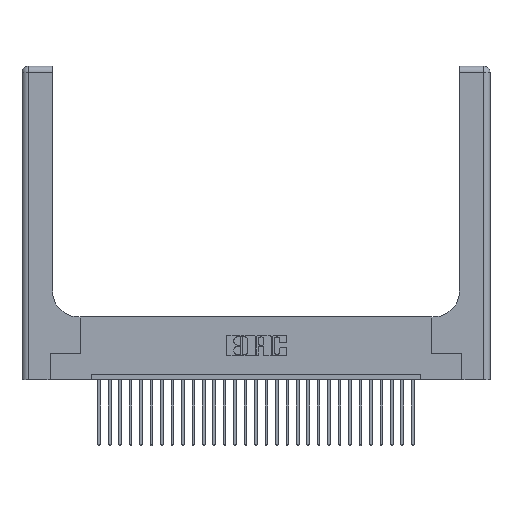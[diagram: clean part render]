
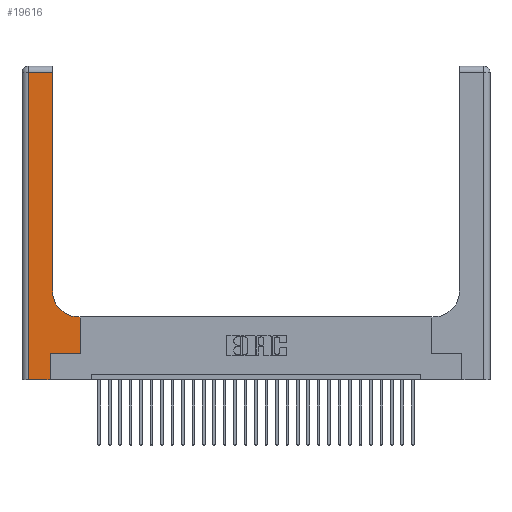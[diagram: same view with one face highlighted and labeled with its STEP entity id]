
A CAD part, top view. The second image highlights one B-rep face of the part: STEP entity #19616.
In plain terms, the highlighted planar face has unit normal (0, 0, 1).
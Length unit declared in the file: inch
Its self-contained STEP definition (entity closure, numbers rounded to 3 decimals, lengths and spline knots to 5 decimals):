
#336 = PLANE ( 'NONE',  #2996 ) ;
#533 = CARTESIAN_POINT ( 'NONE',  ( 0., 3., 0.37 ) ) ;
#578 = VERTEX_POINT ( 'NONE', #17617 ) ;
#620 = FACE_OUTER_BOUND ( 'NONE', #22212, .T. ) ;
#878 = CARTESIAN_POINT ( 'NONE',  ( 0.5585, 0.6, 0.37 ) ) ;
#1505 = DIRECTION ( 'NONE',  ( 0., 1., 0. ) ) ;
#1787 = DIRECTION ( 'NONE',  ( 0., -1., 0. ) ) ;
#2162 = EDGE_CURVE ( 'NONE', #27931, #6418, #3006, .T. ) ;
#2707 = DIRECTION ( 'NONE',  ( 0., 0., -1. ) ) ;
#2772 = CARTESIAN_POINT ( 'NONE',  ( 0.269, 0., 0.37 ) ) ;
#2802 = DIRECTION ( 'NONE',  ( 1., 0., 0. ) ) ;
#2810 = CIRCLE ( 'NONE', #25378, 0.25 ) ;
#2996 = AXIS2_PLACEMENT_3D ( 'NONE', #533, #2707, #21513 ) ;
#3006 = LINE ( 'NONE', #23691, #20864 ) ;
#3022 = CARTESIAN_POINT ( 'NONE',  ( 0.269, 0., 0.37 ) ) ;
#3144 = ORIENTED_EDGE ( 'NONE', *, *, #25434, .T. ) ;
#3261 = EDGE_CURVE ( 'NONE', #21306, #27931, #22228, .T. ) ;
#3919 = LINE ( 'NONE', #5974, #7171 ) ;
#4298 = ORIENTED_EDGE ( 'NONE', *, *, #2162, .T. ) ;
#5940 = ORIENTED_EDGE ( 'NONE', *, *, #27936, .T. ) ;
#5974 = CARTESIAN_POINT ( 'NONE',  ( 0.5585, 0.25, 0.37 ) ) ;
#6418 = VERTEX_POINT ( 'NONE', #29458 ) ;
#7171 = VECTOR ( 'NONE', #1505, 39.37008 ) ;
#8095 = DIRECTION ( 'NONE',  ( 1., 0., 0. ) ) ;
#8713 = ORIENTED_EDGE ( 'NONE', *, *, #9011, .T. ) ;
#9011 = EDGE_CURVE ( 'NONE', #9579, #21306, #2810, .T. ) ;
#9334 = DIRECTION ( 'NONE',  ( 1., 0., 0. ) ) ;
#9579 = VERTEX_POINT ( 'NONE', #21170 ) ;
#9680 = DIRECTION ( 'NONE',  ( 0., 1., 0. ) ) ;
#10049 = ORIENTED_EDGE ( 'NONE', *, *, #25896, .T. ) ;
#11546 = VECTOR ( 'NONE', #9334, 39.37008 ) ;
#14969 = CARTESIAN_POINT ( 'NONE',  ( 0.269, 0.25, 0.37 ) ) ;
#15215 = ORIENTED_EDGE ( 'NONE', *, *, #16431, .T. ) ;
#16431 = EDGE_CURVE ( 'NONE', #18163, #20797, #20680, .T. ) ;
#17021 = VECTOR ( 'NONE', #1787, 39.37008 ) ;
#17460 = DIRECTION ( 'NONE',  ( 0., 1., 0. ) ) ;
#17617 = CARTESIAN_POINT ( 'NONE',  ( 0.06, 0., 0.37 ) ) ;
#17942 = LINE ( 'NONE', #2772, #29420 ) ;
#17976 = CARTESIAN_POINT ( 'NONE',  ( 0.06, 3., 0.37 ) ) ;
#18163 = VERTEX_POINT ( 'NONE', #14969 ) ;
#18689 = CARTESIAN_POINT ( 'NONE',  ( 0.269, 0.25, 0.37 ) ) ;
#18754 = LINE ( 'NONE', #28618, #29914 ) ;
#19616 = ADVANCED_FACE ( 'NONE', ( #620 ), #336, .F. ) ;
#20007 = CARTESIAN_POINT ( 'NONE',  ( 0.5415, 0.85, 0.37 ) ) ;
#20223 = EDGE_CURVE ( 'NONE', #20485, #9579, #29965, .T. ) ;
#20303 = VECTOR ( 'NONE', #20566, 39.37008 ) ;
#20485 = VERTEX_POINT ( 'NONE', #878 ) ;
#20566 = DIRECTION ( 'NONE',  ( -1., 0., 0. ) ) ;
#20680 = LINE ( 'NONE', #18689, #11546 ) ;
#20797 = VERTEX_POINT ( 'NONE', #29850 ) ;
#20864 = VECTOR ( 'NONE', #27919, 39.37008 ) ;
#20972 = VERTEX_POINT ( 'NONE', #3022 ) ;
#21170 = CARTESIAN_POINT ( 'NONE',  ( 0.5415, 0.6, 0.37 ) ) ;
#21306 = VERTEX_POINT ( 'NONE', #26764 ) ;
#21513 = DIRECTION ( 'NONE',  ( -1., 0., 0. ) ) ;
#22088 = LINE ( 'NONE', #17976, #17021 ) ;
#22212 = EDGE_LOOP ( 'NONE', ( #25349, #4298, #27303, #10049, #5940, #15215, #3144, #24890, #8713 ) ) ;
#22228 = LINE ( 'NONE', #22386, #29376 ) ;
#22386 = CARTESIAN_POINT ( 'NONE',  ( 0.2915, 3., 0.37 ) ) ;
#23385 = CARTESIAN_POINT ( 'NONE',  ( 0.2915, 2.94, 0.37 ) ) ;
#23691 = CARTESIAN_POINT ( 'NONE',  ( 0., 2.94, 0.37 ) ) ;
#24457 = EDGE_CURVE ( 'NONE', #6418, #578, #22088, .T. ) ;
#24596 = CARTESIAN_POINT ( 'NONE',  ( 0.2915, 0.6, 0.37 ) ) ;
#24890 = ORIENTED_EDGE ( 'NONE', *, *, #20223, .T. ) ;
#25349 = ORIENTED_EDGE ( 'NONE', *, *, #3261, .T. ) ;
#25378 = AXIS2_PLACEMENT_3D ( 'NONE', #20007, #29111, #8095 ) ;
#25434 = EDGE_CURVE ( 'NONE', #20797, #20485, #3919, .T. ) ;
#25896 = EDGE_CURVE ( 'NONE', #578, #20972, #18754, .T. ) ;
#26764 = CARTESIAN_POINT ( 'NONE',  ( 0.2915, 0.85, 0.37 ) ) ;
#27303 = ORIENTED_EDGE ( 'NONE', *, *, #24457, .T. ) ;
#27919 = DIRECTION ( 'NONE',  ( -1., 0., 0. ) ) ;
#27931 = VERTEX_POINT ( 'NONE', #23385 ) ;
#27936 = EDGE_CURVE ( 'NONE', #20972, #18163, #17942, .T. ) ;
#28618 = CARTESIAN_POINT ( 'NONE',  ( 0., 0., 0.37 ) ) ;
#29111 = DIRECTION ( 'NONE',  ( 0., 0., -1. ) ) ;
#29376 = VECTOR ( 'NONE', #17460, 39.37008 ) ;
#29420 = VECTOR ( 'NONE', #9680, 39.37008 ) ;
#29458 = CARTESIAN_POINT ( 'NONE',  ( 0.06, 2.94, 0.37 ) ) ;
#29850 = CARTESIAN_POINT ( 'NONE',  ( 0.5585, 0.25, 0.37 ) ) ;
#29914 = VECTOR ( 'NONE', #2802, 39.37008 ) ;
#29965 = LINE ( 'NONE', #24596, #20303 ) ;
